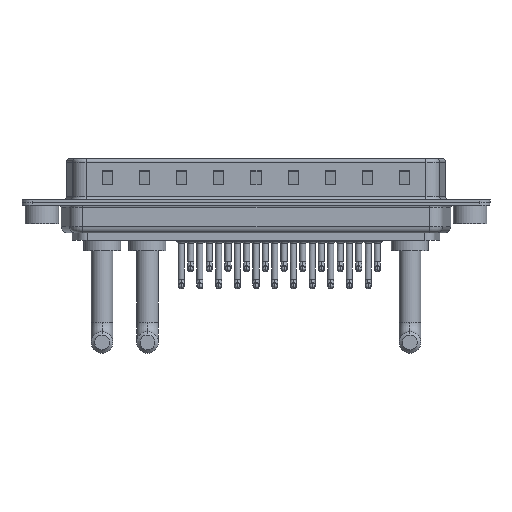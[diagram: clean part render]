
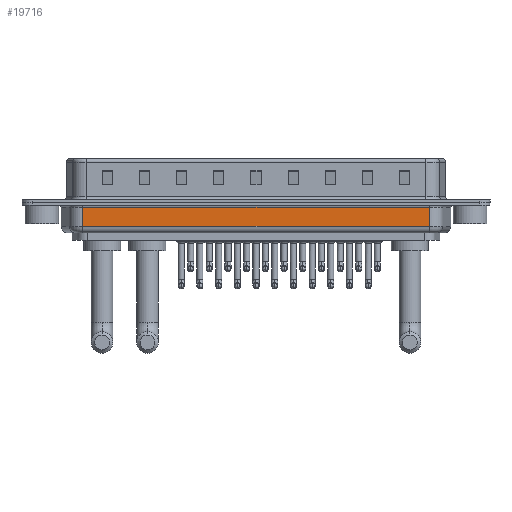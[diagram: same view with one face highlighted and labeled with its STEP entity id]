
A CAD part, front view. The second image highlights one B-rep face of the part: STEP entity #19716.
In plain terms, the highlighted planar face has unit normal (0, -1, 0).
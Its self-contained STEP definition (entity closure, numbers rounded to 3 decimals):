
#1421 = DIRECTION ( 'NONE',  ( 1., 0., 0. ) ) ;
#2060 = VERTEX_POINT ( 'NONE', #8003 ) ;
#3957 = VECTOR ( 'NONE', #1421, 1000. ) ;
#4514 = CARTESIAN_POINT ( 'NONE',  ( 6.031, -5.35, -4.5 ) ) ;
#5077 = CARTESIAN_POINT ( 'NONE',  ( 6.031, -5.35, -0.65 ) ) ;
#5589 = DIRECTION ( 'NONE',  ( -1., 0., 0. ) ) ;
#5946 = CARTESIAN_POINT ( 'NONE',  ( 6.031, -5.35, -0.65 ) ) ;
#6136 = CARTESIAN_POINT ( 'NONE',  ( 57.469, -5.35, -4.5 ) ) ;
#7036 = EDGE_CURVE ( 'NONE', #2060, #26249, #27642, .T. ) ;
#8003 = CARTESIAN_POINT ( 'NONE',  ( 57.469, -5.35, -3.5 ) ) ;
#8068 = DIRECTION ( 'NONE',  ( -1., 0., 0. ) ) ;
#9209 = EDGE_CURVE ( 'NONE', #12406, #2060, #27449, .T. ) ;
#9216 = EDGE_CURVE ( 'NONE', #26249, #10517, #10051, .T. ) ;
#9271 = PLANE ( 'NONE',  #18897 ) ;
#9841 = CARTESIAN_POINT ( 'NONE',  ( 6.031, -5.35, -4.5 ) ) ;
#10051 = LINE ( 'NONE', #5946, #19783 ) ;
#10338 = VECTOR ( 'NONE', #26303, 1000. ) ;
#10429 = EDGE_CURVE ( 'NONE', #12406, #10517, #19957, .T. ) ;
#10517 = VERTEX_POINT ( 'NONE', #5077 ) ;
#11607 = CARTESIAN_POINT ( 'NONE',  ( 57.469, -5.35, -0.65 ) ) ;
#11790 = ORIENTED_EDGE ( 'NONE', *, *, #9209, .T. ) ;
#12406 = VERTEX_POINT ( 'NONE', #18209 ) ;
#14237 = FACE_OUTER_BOUND ( 'NONE', #23821, .T. ) ;
#14633 = ORIENTED_EDGE ( 'NONE', *, *, #7036, .T. ) ;
#15182 = VECTOR ( 'NONE', #19731, 1000. ) ;
#18209 = CARTESIAN_POINT ( 'NONE',  ( 6.031, -5.35, -3.5 ) ) ;
#18897 = AXIS2_PLACEMENT_3D ( 'NONE', #9841, #20467, #5589 ) ;
#19716 = ADVANCED_FACE ( 'NONE', ( #14237 ), #9271, .F. ) ;
#19731 = DIRECTION ( 'NONE',  ( 0., 0., 1. ) ) ;
#19783 = VECTOR ( 'NONE', #8068, 1000. ) ;
#19957 = LINE ( 'NONE', #4514, #10338 ) ;
#20467 = DIRECTION ( 'NONE',  ( 0., 1., 0. ) ) ;
#20836 = CARTESIAN_POINT ( 'NONE',  ( 6.031, -5.35, -3.5 ) ) ;
#21275 = ORIENTED_EDGE ( 'NONE', *, *, #10429, .F. ) ;
#23821 = EDGE_LOOP ( 'NONE', ( #21275, #11790, #14633, #26301 ) ) ;
#26249 = VERTEX_POINT ( 'NONE', #11607 ) ;
#26301 = ORIENTED_EDGE ( 'NONE', *, *, #9216, .T. ) ;
#26303 = DIRECTION ( 'NONE',  ( 0., 0., 1. ) ) ;
#27449 = LINE ( 'NONE', #20836, #3957 ) ;
#27642 = LINE ( 'NONE', #6136, #15182 ) ;
